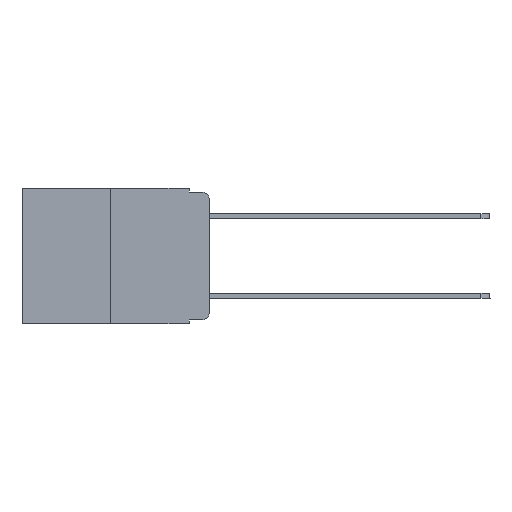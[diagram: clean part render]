
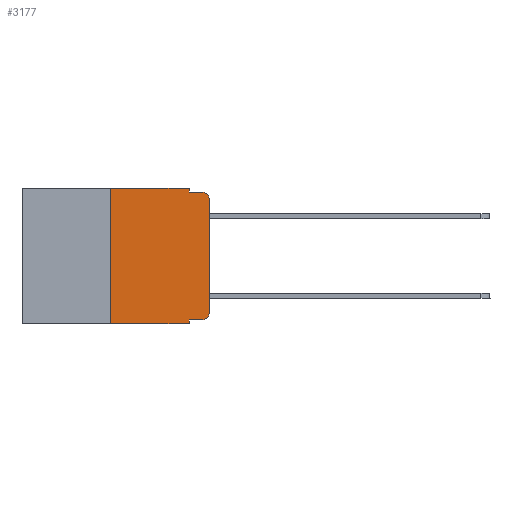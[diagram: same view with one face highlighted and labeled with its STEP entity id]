
A CAD part, left-side view. The second image highlights one B-rep face of the part: STEP entity #3177.
In plain terms, the highlighted planar face has unit normal (-1, 0, 0).
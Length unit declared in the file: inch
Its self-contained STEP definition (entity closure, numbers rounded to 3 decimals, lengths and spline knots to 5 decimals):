
#445 = DIRECTION ( 'NONE',  ( -1., 0., 0. ) ) ;
#530 = VECTOR ( 'NONE', #7742, 39.37008 ) ;
#648 = VECTOR ( 'NONE', #8369, 39.37008 ) ;
#715 = CARTESIAN_POINT ( 'NONE',  ( 0., 0.051, -0.01 ) ) ;
#785 = EDGE_CURVE ( 'NONE', #14711, #6102, #1744, .T. ) ;
#1307 = EDGE_CURVE ( 'NONE', #8384, #8829, #9807, .T. ) ;
#1744 = LINE ( 'NONE', #9160, #10919 ) ;
#1769 = VERTEX_POINT ( 'NONE', #8578 ) ;
#2058 = CIRCLE ( 'NONE', #2165, 0.02 ) ;
#2165 = AXIS2_PLACEMENT_3D ( 'NONE', #12901, #2285, #15078 ) ;
#2248 = DIRECTION ( 'NONE',  ( 0., 0., 1. ) ) ;
#2285 = DIRECTION ( 'NONE',  ( -1., 0., 0. ) ) ;
#2599 = CIRCLE ( 'NONE', #9726, 0.02 ) ;
#2685 = EDGE_CURVE ( 'NONE', #7172, #12105, #7500, .T. ) ;
#3177 = ADVANCED_FACE ( 'NONE', ( #12378 ), #12007, .F. ) ;
#3199 = VECTOR ( 'NONE', #14527, 39.37008 ) ;
#3269 = CARTESIAN_POINT ( 'NONE',  ( 0., 0.02, -0.01 ) ) ;
#3614 = CARTESIAN_POINT ( 'NONE',  ( 0., 0.051, 0. ) ) ;
#3996 = CARTESIAN_POINT ( 'NONE',  ( 0., 0.051, -0.333 ) ) ;
#4091 = EDGE_CURVE ( 'NONE', #14711, #8829, #6963, .T. ) ;
#4467 = VECTOR ( 'NONE', #7818, 39.37008 ) ;
#4547 = ORIENTED_EDGE ( 'NONE', *, *, #7949, .F. ) ;
#4686 = LINE ( 'NONE', #3996, #3199 ) ;
#4755 = CARTESIAN_POINT ( 'NONE',  ( 0., 0.25, 0. ) ) ;
#4968 = CARTESIAN_POINT ( 'NONE',  ( 0., 0., -0.313 ) ) ;
#5162 = DIRECTION ( 'NONE',  ( 0., -1., 0. ) ) ;
#5387 = CARTESIAN_POINT ( 'NONE',  ( 0., 0.051, 0. ) ) ;
#5592 = DIRECTION ( 'NONE',  ( 0., -1., 0. ) ) ;
#5642 = EDGE_LOOP ( 'NONE', ( #10225, #12994, #11273, #14753, #4547, #7438, #6788, #10162, #10952, #6608 ) ) ;
#6102 = VERTEX_POINT ( 'NONE', #4755 ) ;
#6183 = CARTESIAN_POINT ( 'NONE',  ( 0., 0.473, 0. ) ) ;
#6193 = CARTESIAN_POINT ( 'NONE',  ( 0., 0.051, -0.01 ) ) ;
#6463 = DIRECTION ( 'NONE',  ( 0., 0., -1. ) ) ;
#6509 = EDGE_CURVE ( 'NONE', #7771, #1769, #12420, .T. ) ;
#6608 = ORIENTED_EDGE ( 'NONE', *, *, #10141, .T. ) ;
#6788 = ORIENTED_EDGE ( 'NONE', *, *, #4091, .T. ) ;
#6963 = LINE ( 'NONE', #14869, #4467 ) ;
#7172 = VERTEX_POINT ( 'NONE', #6193 ) ;
#7438 = ORIENTED_EDGE ( 'NONE', *, *, #785, .F. ) ;
#7471 = CARTESIAN_POINT ( 'NONE',  ( 0., 0.25, -0.343 ) ) ;
#7500 = LINE ( 'NONE', #715, #13772 ) ;
#7742 = DIRECTION ( 'NONE',  ( 0., 0., 1. ) ) ;
#7744 = LINE ( 'NONE', #11120, #12560 ) ;
#7771 = VERTEX_POINT ( 'NONE', #4968 ) ;
#7818 = DIRECTION ( 'NONE',  ( 0., -1., 0. ) ) ;
#7949 = EDGE_CURVE ( 'NONE', #6102, #14347, #7744, .T. ) ;
#8016 = EDGE_CURVE ( 'NONE', #8384, #13760, #4686, .T. ) ;
#8369 = DIRECTION ( 'NONE',  ( 0., 0., -1. ) ) ;
#8384 = VERTEX_POINT ( 'NONE', #13196 ) ;
#8521 = CARTESIAN_POINT ( 'NONE',  ( 0., 0.02, -0.313 ) ) ;
#8573 = DIRECTION ( 'NONE',  ( 0., 0., -1. ) ) ;
#8578 = CARTESIAN_POINT ( 'NONE',  ( 0., 0., -0.03 ) ) ;
#8829 = VERTEX_POINT ( 'NONE', #11656 ) ;
#9160 = CARTESIAN_POINT ( 'NONE',  ( 0., 0.25, 0. ) ) ;
#9190 = CARTESIAN_POINT ( 'NONE',  ( 0., 0.02, -0.333 ) ) ;
#9726 = AXIS2_PLACEMENT_3D ( 'NONE', #8521, #445, #8573 ) ;
#9807 = LINE ( 'NONE', #3614, #648 ) ;
#10141 = EDGE_CURVE ( 'NONE', #13760, #7771, #2599, .T. ) ;
#10162 = ORIENTED_EDGE ( 'NONE', *, *, #1307, .F. ) ;
#10225 = ORIENTED_EDGE ( 'NONE', *, *, #6509, .T. ) ;
#10500 = LINE ( 'NONE', #5387, #12140 ) ;
#10503 = EDGE_CURVE ( 'NONE', #1769, #12105, #2058, .T. ) ;
#10889 = EDGE_CURVE ( 'NONE', #14347, #7172, #10500, .T. ) ;
#10919 = VECTOR ( 'NONE', #2248, 39.37008 ) ;
#10952 = ORIENTED_EDGE ( 'NONE', *, *, #8016, .T. ) ;
#11120 = CARTESIAN_POINT ( 'NONE',  ( 0., 0.473, 0. ) ) ;
#11273 = ORIENTED_EDGE ( 'NONE', *, *, #2685, .F. ) ;
#11468 = CARTESIAN_POINT ( 'NONE',  ( 0., 0.051, 0. ) ) ;
#11656 = CARTESIAN_POINT ( 'NONE',  ( 0., 0.051, -0.343 ) ) ;
#12007 = PLANE ( 'NONE',  #12519 ) ;
#12105 = VERTEX_POINT ( 'NONE', #3269 ) ;
#12140 = VECTOR ( 'NONE', #6463, 39.37008 ) ;
#12378 = FACE_OUTER_BOUND ( 'NONE', #5642, .T. ) ;
#12420 = LINE ( 'NONE', #13722, #530 ) ;
#12519 = AXIS2_PLACEMENT_3D ( 'NONE', #6183, #13172, #14335 ) ;
#12560 = VECTOR ( 'NONE', #5162, 39.37008 ) ;
#12901 = CARTESIAN_POINT ( 'NONE',  ( 0., 0.02, -0.03 ) ) ;
#12994 = ORIENTED_EDGE ( 'NONE', *, *, #10503, .T. ) ;
#13172 = DIRECTION ( 'NONE',  ( 1., 0., 0. ) ) ;
#13196 = CARTESIAN_POINT ( 'NONE',  ( 0., 0.051, -0.333 ) ) ;
#13722 = CARTESIAN_POINT ( 'NONE',  ( 0., 0., 0. ) ) ;
#13760 = VERTEX_POINT ( 'NONE', #9190 ) ;
#13772 = VECTOR ( 'NONE', #5592, 39.37008 ) ;
#14335 = DIRECTION ( 'NONE',  ( 0., 0., -1. ) ) ;
#14347 = VERTEX_POINT ( 'NONE', #11468 ) ;
#14527 = DIRECTION ( 'NONE',  ( 0., -1., 0. ) ) ;
#14711 = VERTEX_POINT ( 'NONE', #7471 ) ;
#14753 = ORIENTED_EDGE ( 'NONE', *, *, #10889, .F. ) ;
#14869 = CARTESIAN_POINT ( 'NONE',  ( 0., 0.473, -0.343 ) ) ;
#15078 = DIRECTION ( 'NONE',  ( 0., 0., -1. ) ) ;
